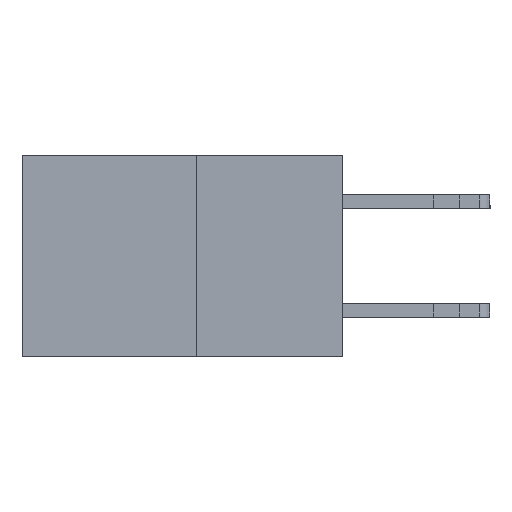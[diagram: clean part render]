
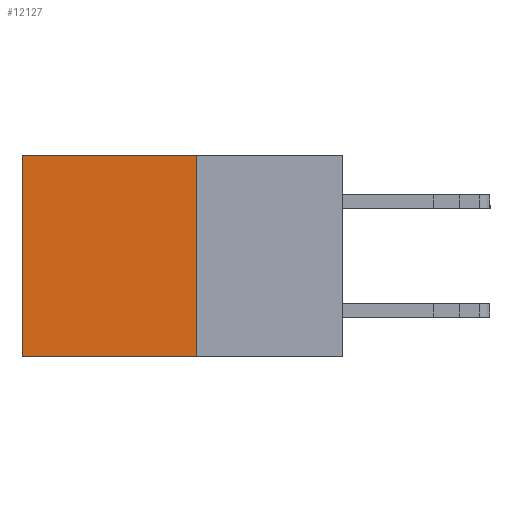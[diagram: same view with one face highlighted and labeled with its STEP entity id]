
A CAD part, left-side view. The second image highlights one B-rep face of the part: STEP entity #12127.
In plain terms, the highlighted planar face has unit normal (-1, 0, 0).
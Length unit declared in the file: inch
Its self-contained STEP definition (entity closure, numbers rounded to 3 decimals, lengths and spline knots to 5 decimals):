
#87 = EDGE_CURVE ( 'NONE', #27600, #20396, #9310, .T. ) ;
#1945 = DIRECTION ( 'NONE',  ( 0., 0., -1. ) ) ;
#2701 = DIRECTION ( 'NONE',  ( 0., 0., -1. ) ) ;
#3768 = AXIS2_PLACEMENT_3D ( 'NONE', #16079, #11042, #28896 ) ;
#5452 = CARTESIAN_POINT ( 'NONE',  ( 0.277, 0.59, 0. ) ) ;
#8454 = PLANE ( 'NONE',  #3768 ) ;
#8464 = ORIENTED_EDGE ( 'NONE', *, *, #87, .F. ) ;
#9310 = LINE ( 'NONE', #21528, #16123 ) ;
#9363 = VERTEX_POINT ( 'NONE', #5452 ) ;
#9586 = ORIENTED_EDGE ( 'NONE', *, *, #32052, .F. ) ;
#10298 = VECTOR ( 'NONE', #2701, 39.37008 ) ;
#11042 = DIRECTION ( 'NONE',  ( 1., 0., 0. ) ) ;
#11799 = VECTOR ( 'NONE', #17930, 39.37008 ) ;
#12127 = ADVANCED_FACE ( 'NONE', ( #19948 ), #8454, .F. ) ;
#12186 = ORIENTED_EDGE ( 'NONE', *, *, #21549, .T. ) ;
#13757 = EDGE_CURVE ( 'NONE', #27600, #9363, #31252, .T. ) ;
#14555 = CARTESIAN_POINT ( 'NONE',  ( 0.277, 0.27, 0. ) ) ;
#15409 = CARTESIAN_POINT ( 'NONE',  ( 0.277, 0.59, -0.37 ) ) ;
#15789 = EDGE_LOOP ( 'NONE', ( #12186, #9586, #8464, #18109 ) ) ;
#16079 = CARTESIAN_POINT ( 'NONE',  ( 0.277, 0.27, -0.37 ) ) ;
#16123 = VECTOR ( 'NONE', #1945, 39.37008 ) ;
#16950 = VECTOR ( 'NONE', #18932, 39.37008 ) ;
#17126 = LINE ( 'NONE', #15409, #10298 ) ;
#17774 = LINE ( 'NONE', #31507, #16950 ) ;
#17930 = DIRECTION ( 'NONE',  ( 0., 1., 0. ) ) ;
#18109 = ORIENTED_EDGE ( 'NONE', *, *, #13757, .T. ) ;
#18932 = DIRECTION ( 'NONE',  ( 0., 1., 0. ) ) ;
#18975 = CARTESIAN_POINT ( 'NONE',  ( 0.277, 0.27, -0.37 ) ) ;
#19948 = FACE_OUTER_BOUND ( 'NONE', #15789, .T. ) ;
#20396 = VERTEX_POINT ( 'NONE', #18975 ) ;
#21528 = CARTESIAN_POINT ( 'NONE',  ( 0.277, 0.27, -0.37 ) ) ;
#21549 = EDGE_CURVE ( 'NONE', #9363, #29822, #17126, .T. ) ;
#27600 = VERTEX_POINT ( 'NONE', #14555 ) ;
#28896 = DIRECTION ( 'NONE',  ( 0., 0., -1. ) ) ;
#29043 = CARTESIAN_POINT ( 'NONE',  ( 0.277, 0.59, -0.37 ) ) ;
#29822 = VERTEX_POINT ( 'NONE', #29043 ) ;
#30183 = CARTESIAN_POINT ( 'NONE',  ( 0.277, 0.27, 0. ) ) ;
#31252 = LINE ( 'NONE', #30183, #11799 ) ;
#31507 = CARTESIAN_POINT ( 'NONE',  ( 0.277, 0.27, -0.37 ) ) ;
#32052 = EDGE_CURVE ( 'NONE', #20396, #29822, #17774, .T. ) ;
